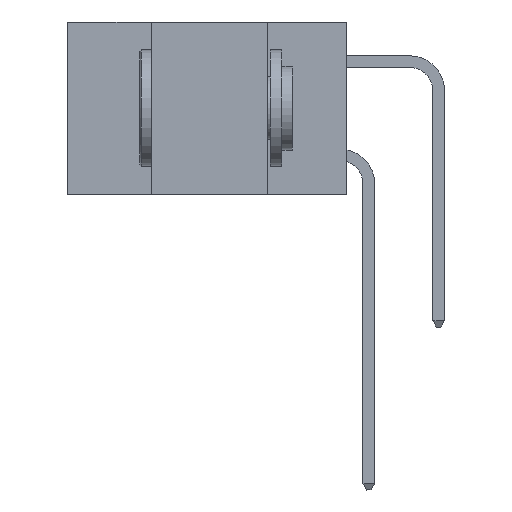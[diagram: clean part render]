
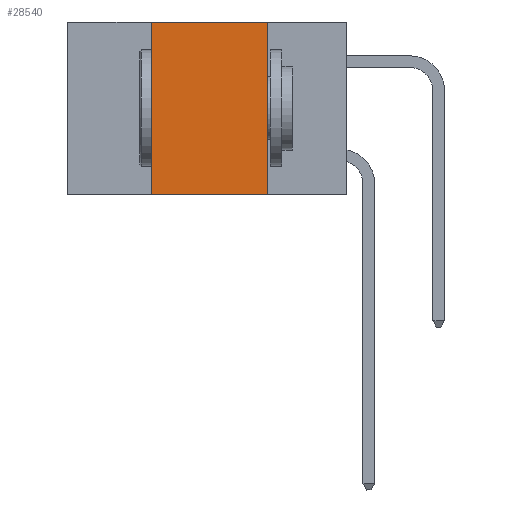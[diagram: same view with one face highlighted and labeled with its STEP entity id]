
A CAD part, left-side view. The second image highlights one B-rep face of the part: STEP entity #28540.
In plain terms, the highlighted planar face has unit normal (-1, 0, 0).
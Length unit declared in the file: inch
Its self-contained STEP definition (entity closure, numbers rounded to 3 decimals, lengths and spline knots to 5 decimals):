
#1194 = CARTESIAN_POINT ( 'NONE',  ( 0., 0.6, 0. ) ) ;
#2264 = FACE_OUTER_BOUND ( 'NONE', #32910, .T. ) ;
#2514 = EDGE_CURVE ( 'NONE', #33996, #43327, #2521, .T. ) ;
#2521 = LINE ( 'NONE', #30445, #5844 ) ;
#2630 = CARTESIAN_POINT ( 'NONE',  ( 0., 0.6, -0.37 ) ) ;
#4526 = LINE ( 'NONE', #13767, #23335 ) ;
#4818 = EDGE_CURVE ( 'NONE', #44783, #10024, #4526, .T. ) ;
#4915 = ORIENTED_EDGE ( 'NONE', *, *, #44737, .F. ) ;
#5844 = VECTOR ( 'NONE', #19907, 39.37008 ) ;
#7225 = LINE ( 'NONE', #2630, #43160 ) ;
#8527 = ORIENTED_EDGE ( 'NONE', *, *, #2514, .F. ) ;
#10024 = VERTEX_POINT ( 'NONE', #20556 ) ;
#12955 = VECTOR ( 'NONE', #23271, 39.37008 ) ;
#13065 = PLANE ( 'NONE',  #17617 ) ;
#13767 = CARTESIAN_POINT ( 'NONE',  ( 0., 0.42, 0. ) ) ;
#16634 = CARTESIAN_POINT ( 'NONE',  ( 0., 0.6, 0. ) ) ;
#17617 = AXIS2_PLACEMENT_3D ( 'NONE', #16634, #41308, #44867 ) ;
#19907 = DIRECTION ( 'NONE',  ( 0., 0., -1. ) ) ;
#20556 = CARTESIAN_POINT ( 'NONE',  ( 0., 0.42, 0. ) ) ;
#23271 = DIRECTION ( 'NONE',  ( 0., -1., 0. ) ) ;
#23335 = VECTOR ( 'NONE', #24424, 39.37008 ) ;
#23953 = DIRECTION ( 'NONE',  ( 0., -1., 0. ) ) ;
#24424 = DIRECTION ( 'NONE',  ( 0., 0., 1. ) ) ;
#24511 = EDGE_CURVE ( 'NONE', #44783, #43327, #7225, .T. ) ;
#28540 = ADVANCED_FACE ( 'NONE', ( #2264 ), #13065, .F. ) ;
#30445 = CARTESIAN_POINT ( 'NONE',  ( 0., 0.17, 0. ) ) ;
#32910 = EDGE_LOOP ( 'NONE', ( #8527, #4915, #34074, #42928 ) ) ;
#33996 = VERTEX_POINT ( 'NONE', #38384 ) ;
#34074 = ORIENTED_EDGE ( 'NONE', *, *, #4818, .F. ) ;
#35045 = LINE ( 'NONE', #1194, #12955 ) ;
#38384 = CARTESIAN_POINT ( 'NONE',  ( 0., 0.17, 0. ) ) ;
#39615 = CARTESIAN_POINT ( 'NONE',  ( 0., 0.17, -0.37 ) ) ;
#41308 = DIRECTION ( 'NONE',  ( 1., 0., 0. ) ) ;
#42928 = ORIENTED_EDGE ( 'NONE', *, *, #24511, .T. ) ;
#43160 = VECTOR ( 'NONE', #23953, 39.37008 ) ;
#43327 = VERTEX_POINT ( 'NONE', #39615 ) ;
#44727 = CARTESIAN_POINT ( 'NONE',  ( 0., 0.42, -0.37 ) ) ;
#44737 = EDGE_CURVE ( 'NONE', #10024, #33996, #35045, .T. ) ;
#44783 = VERTEX_POINT ( 'NONE', #44727 ) ;
#44867 = DIRECTION ( 'NONE',  ( 0., 0., -1. ) ) ;
